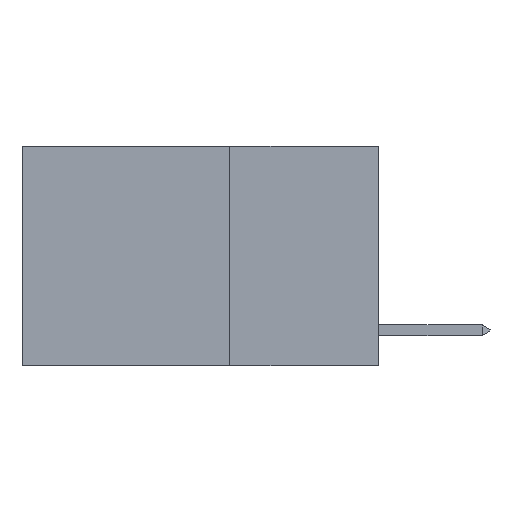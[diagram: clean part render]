
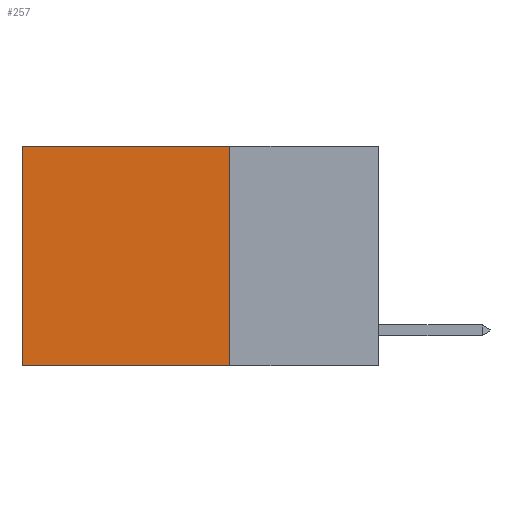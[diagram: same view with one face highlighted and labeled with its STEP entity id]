
A CAD part, left-side view. The second image highlights one B-rep face of the part: STEP entity #257.
In plain terms, the highlighted planar face has unit normal (-1, 0, 0).
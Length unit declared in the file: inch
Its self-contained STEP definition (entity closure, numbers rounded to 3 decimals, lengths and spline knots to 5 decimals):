
#257 = ADVANCED_FACE ( 'NONE', ( #6582 ), #5793, .F. ) ;
#311 = EDGE_CURVE ( 'NONE', #3113, #5134, #8378, .T. ) ;
#325 = AXIS2_PLACEMENT_3D ( 'NONE', #5845, #8132, #9692 ) ;
#351 = VERTEX_POINT ( 'NONE', #3068 ) ;
#723 = EDGE_CURVE ( 'NONE', #351, #8806, #2374, .T. ) ;
#1072 = CARTESIAN_POINT ( 'NONE',  ( 0.2625, 0.25, 0. ) ) ;
#1384 = CARTESIAN_POINT ( 'NONE',  ( 0.2625, 0.25, 0. ) ) ;
#1743 = LINE ( 'NONE', #1072, #3519 ) ;
#2374 = LINE ( 'NONE', #7707, #7350 ) ;
#2428 = VECTOR ( 'NONE', #9957, 39.37008 ) ;
#3039 = DIRECTION ( 'NONE',  ( 0., 1., 0. ) ) ;
#3059 = VECTOR ( 'NONE', #5995, 39.37008 ) ;
#3068 = CARTESIAN_POINT ( 'NONE',  ( 0.2625, 0.25, -0.37 ) ) ;
#3113 = VERTEX_POINT ( 'NONE', #8848 ) ;
#3283 = EDGE_CURVE ( 'NONE', #3113, #351, #1743, .T. ) ;
#3519 = VECTOR ( 'NONE', #7216, 39.37008 ) ;
#4320 = CARTESIAN_POINT ( 'NONE',  ( 0.2625, 0.6, 0. ) ) ;
#5134 = VERTEX_POINT ( 'NONE', #7981 ) ;
#5793 = PLANE ( 'NONE',  #325 ) ;
#5845 = CARTESIAN_POINT ( 'NONE',  ( 0.2625, 0.25, 0. ) ) ;
#5995 = DIRECTION ( 'NONE',  ( 0., 0., -1. ) ) ;
#6571 = ORIENTED_EDGE ( 'NONE', *, *, #3283, .F. ) ;
#6582 = FACE_OUTER_BOUND ( 'NONE', #9257, .T. ) ;
#6629 = LINE ( 'NONE', #4320, #3059 ) ;
#6959 = ORIENTED_EDGE ( 'NONE', *, *, #8745, .T. ) ;
#7216 = DIRECTION ( 'NONE',  ( 0., 0., -1. ) ) ;
#7350 = VECTOR ( 'NONE', #3039, 39.37008 ) ;
#7707 = CARTESIAN_POINT ( 'NONE',  ( 0.2625, 0.25, -0.37 ) ) ;
#7981 = CARTESIAN_POINT ( 'NONE',  ( 0.2625, 0.6, 0. ) ) ;
#8132 = DIRECTION ( 'NONE',  ( 1., 0., 0. ) ) ;
#8378 = LINE ( 'NONE', #1384, #2428 ) ;
#8565 = ORIENTED_EDGE ( 'NONE', *, *, #723, .F. ) ;
#8745 = EDGE_CURVE ( 'NONE', #5134, #8806, #6629, .T. ) ;
#8806 = VERTEX_POINT ( 'NONE', #9943 ) ;
#8848 = CARTESIAN_POINT ( 'NONE',  ( 0.2625, 0.25, 0. ) ) ;
#8881 = ORIENTED_EDGE ( 'NONE', *, *, #311, .T. ) ;
#9257 = EDGE_LOOP ( 'NONE', ( #6959, #8565, #6571, #8881 ) ) ;
#9692 = DIRECTION ( 'NONE',  ( 0., 0., -1. ) ) ;
#9943 = CARTESIAN_POINT ( 'NONE',  ( 0.2625, 0.6, -0.37 ) ) ;
#9957 = DIRECTION ( 'NONE',  ( 0., 1., 0. ) ) ;
